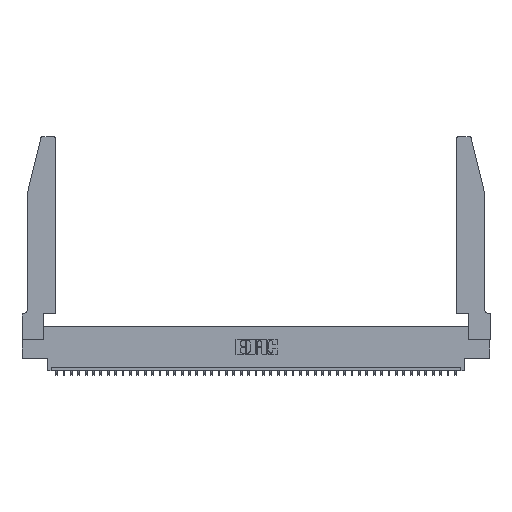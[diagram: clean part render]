
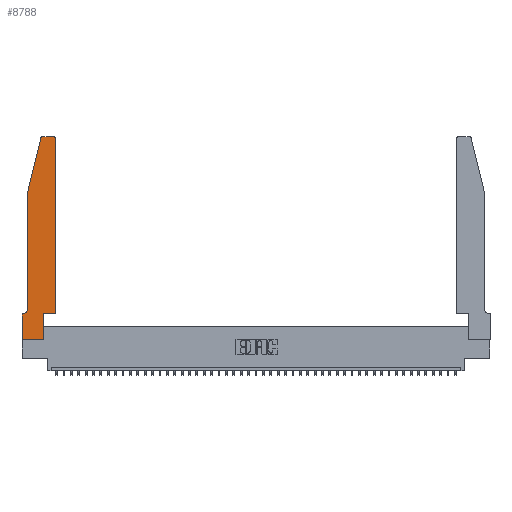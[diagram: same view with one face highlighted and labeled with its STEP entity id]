
A CAD part, top view. The second image highlights one B-rep face of the part: STEP entity #8788.
In plain terms, the highlighted planar face has unit normal (0, 0, 1).
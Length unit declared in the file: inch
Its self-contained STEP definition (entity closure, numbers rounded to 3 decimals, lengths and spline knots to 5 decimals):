
#154 = ORIENTED_EDGE ( 'NONE', *, *, #582, .T. ) ;
#203 = AXIS2_PLACEMENT_3D ( 'NONE', #10337, #10476, #37885 ) ;
#250 = VECTOR ( 'NONE', #5279, 39.37008 ) ;
#582 = EDGE_CURVE ( 'NONE', #23813, #18811, #39110, .T. ) ;
#863 = EDGE_CURVE ( 'NONE', #24898, #16759, #28280, .T. ) ;
#1797 = EDGE_CURVE ( 'NONE', #12924, #5505, #32502, .T. ) ;
#2364 = DIRECTION ( 'NONE',  ( 0., -1., 0. ) ) ;
#2494 = DIRECTION ( 'NONE',  ( 0., 0., 1. ) ) ;
#2688 = CARTESIAN_POINT ( 'NONE',  ( 0.4505, 0.35, 0.37 ) ) ;
#3251 = ORIENTED_EDGE ( 'NONE', *, *, #17451, .T. ) ;
#3281 = VECTOR ( 'NONE', #34370, 39.37008 ) ;
#3304 = VECTOR ( 'NONE', #30432, 39.37008 ) ;
#4048 = CIRCLE ( 'NONE', #30068, 0.03 ) ;
#4209 = CARTESIAN_POINT ( 'NONE',  ( 0.284, 2.75, 0.37 ) ) ;
#5279 = DIRECTION ( 'NONE',  ( 0., 1., 0. ) ) ;
#5325 = EDGE_CURVE ( 'NONE', #19317, #12094, #16153, .T. ) ;
#5505 = VERTEX_POINT ( 'NONE', #23657 ) ;
#5767 = DIRECTION ( 'NONE',  ( 1., 0., 0. ) ) ;
#6829 = VECTOR ( 'NONE', #7767, 39.37008 ) ;
#7344 = CARTESIAN_POINT ( 'NONE',  ( 0.2605, 2.75, 0.37 ) ) ;
#7660 = DIRECTION ( 'NONE',  ( -1., 0., 0. ) ) ;
#7767 = DIRECTION ( 'NONE',  ( 1., 0., 0. ) ) ;
#7882 = CARTESIAN_POINT ( 'NONE',  ( 0.4505, 2.72, 0.37 ) ) ;
#7964 = CARTESIAN_POINT ( 'NONE',  ( 0., 0.35, 0.37 ) ) ;
#8788 = ADVANCED_FACE ( 'NONE', ( #34168 ), #12771, .T. ) ;
#9536 = CARTESIAN_POINT ( 'NONE',  ( 0.284, 2.72, 0.37 ) ) ;
#10147 = CARTESIAN_POINT ( 'NONE',  ( 0.0755, 0.35, 0.37 ) ) ;
#10337 = CARTESIAN_POINT ( 'NONE',  ( 0.4205, 2.72, 0.37 ) ) ;
#10476 = DIRECTION ( 'NONE',  ( 0., 0., 1. ) ) ;
#10556 = CARTESIAN_POINT ( 'NONE',  ( 0.2865, 0., 0.37 ) ) ;
#10585 = EDGE_CURVE ( 'NONE', #30720, #12924, #16251, .T. ) ;
#12094 = VERTEX_POINT ( 'NONE', #4209 ) ;
#12355 = EDGE_CURVE ( 'NONE', #16759, #16020, #34694, .T. ) ;
#12598 = VECTOR ( 'NONE', #13849, 39.37008 ) ;
#12675 = CARTESIAN_POINT ( 'NONE',  ( 0., 0., 0.37 ) ) ;
#12771 = PLANE ( 'NONE',  #24890 ) ;
#12774 = LINE ( 'NONE', #30584, #34339 ) ;
#12843 = CARTESIAN_POINT ( 'NONE',  ( 0.4505, 0.35, 0.37 ) ) ;
#12924 = VERTEX_POINT ( 'NONE', #7964 ) ;
#13382 = CARTESIAN_POINT ( 'NONE',  ( 0., 0.35, 0.37 ) ) ;
#13413 = ORIENTED_EDGE ( 'NONE', *, *, #37280, .T. ) ;
#13849 = DIRECTION ( 'NONE',  ( 0., -1., 0. ) ) ;
#14106 = DIRECTION ( 'NONE',  ( 0., 0., -1. ) ) ;
#14385 = EDGE_CURVE ( 'NONE', #16020, #30720, #33451, .T. ) ;
#14412 = ORIENTED_EDGE ( 'NONE', *, *, #14385, .T. ) ;
#16020 = VERTEX_POINT ( 'NONE', #31365 ) ;
#16153 = LINE ( 'NONE', #7344, #23125 ) ;
#16251 = LINE ( 'NONE', #10147, #3281 ) ;
#16759 = VERTEX_POINT ( 'NONE', #22081 ) ;
#17451 = EDGE_CURVE ( 'NONE', #5505, #43939, #42867, .T. ) ;
#18209 = VERTEX_POINT ( 'NONE', #42092 ) ;
#18811 = VERTEX_POINT ( 'NONE', #7882 ) ;
#19317 = VERTEX_POINT ( 'NONE', #31148 ) ;
#21190 = ORIENTED_EDGE ( 'NONE', *, *, #10585, .T. ) ;
#21414 = ORIENTED_EDGE ( 'NONE', *, *, #863, .T. ) ;
#22081 = CARTESIAN_POINT ( 'NONE',  ( 0.0755, 2., 0.37 ) ) ;
#22699 = LINE ( 'NONE', #12843, #3304 ) ;
#22795 = DIRECTION ( 'NONE',  ( -0.239, -0.971, 0. ) ) ;
#22887 = CARTESIAN_POINT ( 'NONE',  ( 0.0055, 0.35, 0.37 ) ) ;
#23125 = VECTOR ( 'NONE', #7660, 39.37008 ) ;
#23528 = AXIS2_PLACEMENT_3D ( 'NONE', #38170, #14106, #41613 ) ;
#23657 = CARTESIAN_POINT ( 'NONE',  ( 0., 0., 0.37 ) ) ;
#23813 = VERTEX_POINT ( 'NONE', #2688 ) ;
#24305 = CARTESIAN_POINT ( 'NONE',  ( 0.25487, 2.72718, 0.37 ) ) ;
#24890 = AXIS2_PLACEMENT_3D ( 'NONE', #13382, #2494, #30078 ) ;
#24898 = VERTEX_POINT ( 'NONE', #24305 ) ;
#25490 = CARTESIAN_POINT ( 'NONE',  ( 0.4505, 0.35, 0.37 ) ) ;
#26644 = CARTESIAN_POINT ( 'NONE',  ( 0.0755, 2., 0.37 ) ) ;
#26913 = ORIENTED_EDGE ( 'NONE', *, *, #5325, .T. ) ;
#28280 = LINE ( 'NONE', #33464, #34732 ) ;
#29483 = EDGE_LOOP ( 'NONE', ( #26913, #43242, #21414, #33397, #14412, #21190, #30094, #3251, #40523, #13413, #154, #30699 ) ) ;
#30068 = AXIS2_PLACEMENT_3D ( 'NONE', #9536, #33485, #5767 ) ;
#30078 = DIRECTION ( 'NONE',  ( 1., 0., 0. ) ) ;
#30094 = ORIENTED_EDGE ( 'NONE', *, *, #1797, .T. ) ;
#30432 = DIRECTION ( 'NONE',  ( 1., 0., 0. ) ) ;
#30584 = CARTESIAN_POINT ( 'NONE',  ( 0.2865, 0.35, 0.37 ) ) ;
#30699 = ORIENTED_EDGE ( 'NONE', *, *, #37777, .T. ) ;
#30720 = VERTEX_POINT ( 'NONE', #22887 ) ;
#31148 = CARTESIAN_POINT ( 'NONE',  ( 0.4205, 2.75, 0.37 ) ) ;
#31365 = CARTESIAN_POINT ( 'NONE',  ( 0.0755, 0.42, 0.37 ) ) ;
#32194 = CARTESIAN_POINT ( 'NONE',  ( 0., 0., 0.37 ) ) ;
#32502 = LINE ( 'NONE', #12675, #12598 ) ;
#33397 = ORIENTED_EDGE ( 'NONE', *, *, #12355, .T. ) ;
#33451 = CIRCLE ( 'NONE', #23528, 0.07 ) ;
#33464 = CARTESIAN_POINT ( 'NONE',  ( 0.0755, 2., 0.37 ) ) ;
#33485 = DIRECTION ( 'NONE',  ( 0., 0., 1. ) ) ;
#34035 = DIRECTION ( 'NONE',  ( 0., 1., 0. ) ) ;
#34168 = FACE_OUTER_BOUND ( 'NONE', #29483, .T. ) ;
#34190 = VECTOR ( 'NONE', #2364, 39.37008 ) ;
#34339 = VECTOR ( 'NONE', #34035, 39.37008 ) ;
#34370 = DIRECTION ( 'NONE',  ( -1., 0., 0. ) ) ;
#34694 = LINE ( 'NONE', #26644, #34190 ) ;
#34732 = VECTOR ( 'NONE', #22795, 39.37008 ) ;
#37280 = EDGE_CURVE ( 'NONE', #18209, #23813, #22699, .T. ) ;
#37777 = EDGE_CURVE ( 'NONE', #18811, #19317, #38160, .T. ) ;
#37885 = DIRECTION ( 'NONE',  ( 1., 0., 0. ) ) ;
#38160 = CIRCLE ( 'NONE', #203, 0.03 ) ;
#38170 = CARTESIAN_POINT ( 'NONE',  ( 0.0055, 0.42, 0.37 ) ) ;
#38911 = EDGE_CURVE ( 'NONE', #12094, #24898, #4048, .T. ) ;
#39110 = LINE ( 'NONE', #25490, #250 ) ;
#40523 = ORIENTED_EDGE ( 'NONE', *, *, #44506, .T. ) ;
#41613 = DIRECTION ( 'NONE',  ( -1., 0., 0. ) ) ;
#42092 = CARTESIAN_POINT ( 'NONE',  ( 0.2865, 0.35, 0.37 ) ) ;
#42867 = LINE ( 'NONE', #32194, #6829 ) ;
#43242 = ORIENTED_EDGE ( 'NONE', *, *, #38911, .T. ) ;
#43939 = VERTEX_POINT ( 'NONE', #10556 ) ;
#44506 = EDGE_CURVE ( 'NONE', #43939, #18209, #12774, .T. ) ;
